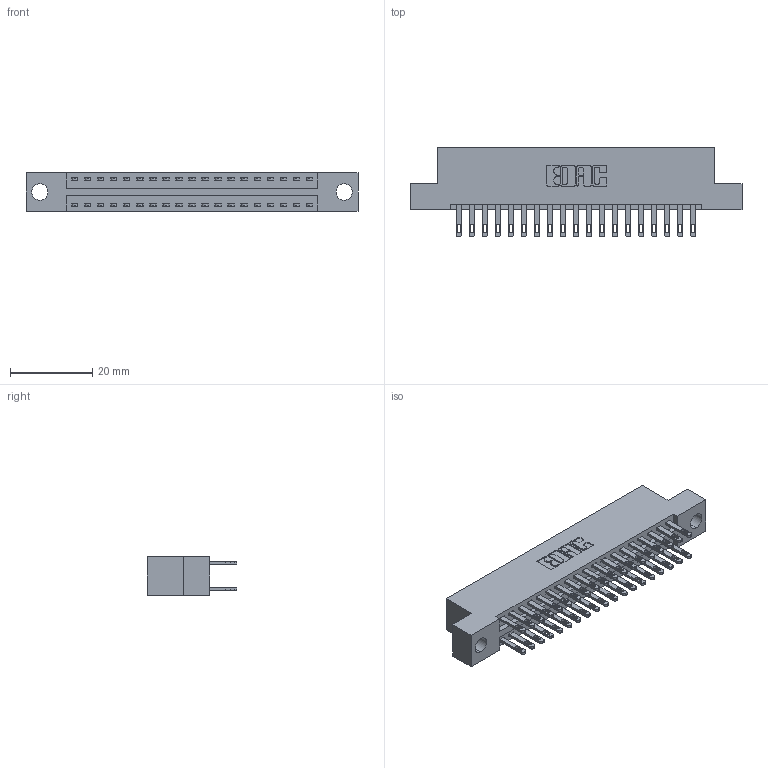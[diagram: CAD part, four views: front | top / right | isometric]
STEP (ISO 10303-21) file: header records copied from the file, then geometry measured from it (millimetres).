
FILE_DESCRIPTION (( 'STEP AP203' ), '1' );
FILE_NAME ('346-038-500-204.STEP', '2022-05-19T22:47:59', ( '' ), ( '' ), 'SwSTEP 2.0', 'SolidWorks 2020', '' );
FILE_SCHEMA (( 'CONFIG_CONTROL_DESIGN' ));
Length unit declared in the file: inch
Products named in the file (3): 346 Part_Flush Mounting Lugs - 0.156 Dia-TH; 345-292-001_345-293-100; 346-038-500-204
Assembly tree (39 placements, depth 2):
  346-038-500-204
    346 Part_Flush Mounting Lugs - 0.156 Dia-TH
    345-292-001_345-293-100  x38
Bounding box: 80.9 x 21.84 x 9.4 mm (x, y, z)
Volume: 7720.2 mm3; surface area: 10496 mm2
Topology: 39 solids, 39 shells, 1960 faces, 5951 edges, 3966 vertices
Faces by surface type: plane 1192, cylinder 768
Entity records: 15845 total; most frequent: CARTESIAN_POINT 2646, ORIENTED_EDGE 2578, DIRECTION 2385, EDGE_CURVE 1289, VECTOR 1077, LINE 1077, VERTEX_POINT 858, AXIS2_PLACEMENT_3D 654
